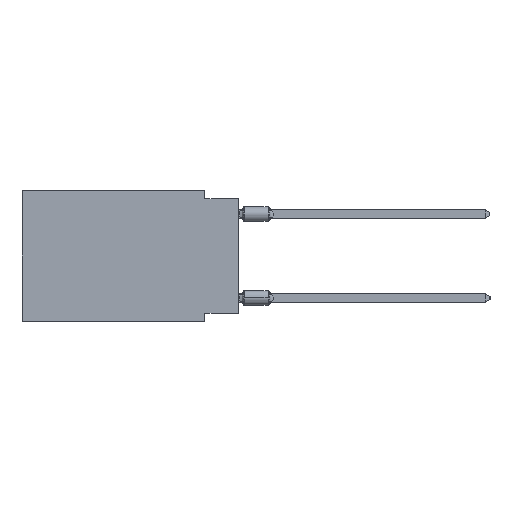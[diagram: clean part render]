
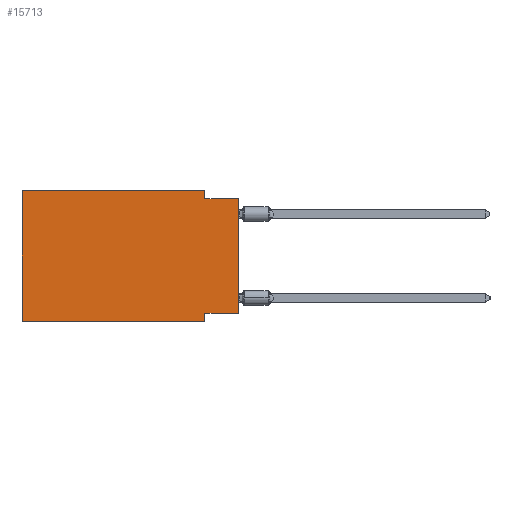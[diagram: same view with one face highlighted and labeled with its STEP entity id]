
A CAD part, left-side view. The second image highlights one B-rep face of the part: STEP entity #15713.
In plain terms, the highlighted planar face has unit normal (-1, 0, 0).
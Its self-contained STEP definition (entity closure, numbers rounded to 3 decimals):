
#450 = EDGE_LOOP ( 'NONE', ( #25573, #35895, #46807, #59695, #64328, #60476, #3902, #8983 ) ) ;
#729 = FACE_OUTER_BOUND ( 'NONE', #450, .T. ) ;
#3515 = AXIS2_PLACEMENT_3D ( 'NONE', #11527, #61065, #20071 ) ;
#3902 = ORIENTED_EDGE ( 'NONE', *, *, #33945, .F. ) ;
#5538 = EDGE_CURVE ( 'NONE', #30922, #60669, #16134, .T. ) ;
#8840 = CARTESIAN_POINT ( 'NONE',  ( 0., 2.54, 0. ) ) ;
#8983 = ORIENTED_EDGE ( 'NONE', *, *, #52530, .F. ) ;
#10487 = VECTOR ( 'NONE', #13177, 1000. ) ;
#11024 = CARTESIAN_POINT ( 'NONE',  ( 0., 16.383, 0. ) ) ;
#11330 = VECTOR ( 'NONE', #32736, 1000. ) ;
#11527 = CARTESIAN_POINT ( 'NONE',  ( 0., 16.383, 0. ) ) ;
#11602 = VERTEX_POINT ( 'NONE', #43726 ) ;
#11729 = LINE ( 'NONE', #26783, #11330 ) ;
#13177 = DIRECTION ( 'NONE',  ( 0., -1., 0. ) ) ;
#13255 = VECTOR ( 'NONE', #61731, 1000. ) ;
#13838 = DIRECTION ( 'NONE',  ( 0., 0., 1. ) ) ;
#14275 = CARTESIAN_POINT ( 'NONE',  ( 0., 2.54, 0. ) ) ;
#15638 = CARTESIAN_POINT ( 'NONE',  ( 0., 2.54, -9.271 ) ) ;
#15713 = ADVANCED_FACE ( 'NONE', ( #729 ), #56473, .F. ) ;
#16100 = DIRECTION ( 'NONE',  ( 0., 1., 0. ) ) ;
#16134 = LINE ( 'NONE', #50898, #13255 ) ;
#18189 = DIRECTION ( 'NONE',  ( 0., -1., 0. ) ) ;
#18984 = LINE ( 'NONE', #8840, #50353 ) ;
#20071 = DIRECTION ( 'NONE',  ( 0., 0., -1. ) ) ;
#20559 = VECTOR ( 'NONE', #16100, 1000. ) ;
#25573 = ORIENTED_EDGE ( 'NONE', *, *, #27191, .T. ) ;
#26417 = CARTESIAN_POINT ( 'NONE',  ( 0., 0., -0.635 ) ) ;
#26783 = CARTESIAN_POINT ( 'NONE',  ( 0., 16.383, 0. ) ) ;
#27191 = EDGE_CURVE ( 'NONE', #29112, #50223, #32538, .T. ) ;
#27917 = LINE ( 'NONE', #46967, #10487 ) ;
#29112 = VERTEX_POINT ( 'NONE', #52447 ) ;
#30400 = VERTEX_POINT ( 'NONE', #49789 ) ;
#30922 = VERTEX_POINT ( 'NONE', #11024 ) ;
#32538 = LINE ( 'NONE', #32864, #53435 ) ;
#32736 = DIRECTION ( 'NONE',  ( 0., 0., 1. ) ) ;
#32851 = EDGE_CURVE ( 'NONE', #30400, #50223, #43091, .T. ) ;
#32864 = CARTESIAN_POINT ( 'NONE',  ( 0., 0., 0. ) ) ;
#33945 = EDGE_CURVE ( 'NONE', #54460, #58143, #37863, .T. ) ;
#35121 = EDGE_CURVE ( 'NONE', #11602, #30922, #11729, .T. ) ;
#35895 = ORIENTED_EDGE ( 'NONE', *, *, #32851, .F. ) ;
#37636 = EDGE_CURVE ( 'NONE', #11602, #58143, #27917, .T. ) ;
#37863 = LINE ( 'NONE', #56621, #49048 ) ;
#38161 = EDGE_CURVE ( 'NONE', #60669, #30400, #18984, .T. ) ;
#42136 = DIRECTION ( 'NONE',  ( 0., 0., -1. ) ) ;
#43091 = LINE ( 'NONE', #63142, #62609 ) ;
#43726 = CARTESIAN_POINT ( 'NONE',  ( 0., 16.383, -9.906 ) ) ;
#46807 = ORIENTED_EDGE ( 'NONE', *, *, #38161, .F. ) ;
#46967 = CARTESIAN_POINT ( 'NONE',  ( 0., 16.383, -9.906 ) ) ;
#49048 = VECTOR ( 'NONE', #42136, 1000. ) ;
#49151 = DIRECTION ( 'NONE',  ( 0., 0., -1. ) ) ;
#49785 = CARTESIAN_POINT ( 'NONE',  ( 0., 2.54, -9.906 ) ) ;
#49789 = CARTESIAN_POINT ( 'NONE',  ( 0., 2.54, -0.635 ) ) ;
#50223 = VERTEX_POINT ( 'NONE', #26417 ) ;
#50353 = VECTOR ( 'NONE', #49151, 1000. ) ;
#50898 = CARTESIAN_POINT ( 'NONE',  ( 0., 16.383, 0. ) ) ;
#52447 = CARTESIAN_POINT ( 'NONE',  ( 0., 0., -9.271 ) ) ;
#52480 = CARTESIAN_POINT ( 'NONE',  ( 0., 0., -9.271 ) ) ;
#52530 = EDGE_CURVE ( 'NONE', #29112, #54460, #61380, .T. ) ;
#53435 = VECTOR ( 'NONE', #13838, 1000. ) ;
#54460 = VERTEX_POINT ( 'NONE', #15638 ) ;
#56473 = PLANE ( 'NONE',  #3515 ) ;
#56621 = CARTESIAN_POINT ( 'NONE',  ( 0., 2.54, -9.906 ) ) ;
#58143 = VERTEX_POINT ( 'NONE', #49785 ) ;
#59695 = ORIENTED_EDGE ( 'NONE', *, *, #5538, .F. ) ;
#60476 = ORIENTED_EDGE ( 'NONE', *, *, #37636, .T. ) ;
#60669 = VERTEX_POINT ( 'NONE', #14275 ) ;
#61065 = DIRECTION ( 'NONE',  ( 1., 0., 0. ) ) ;
#61380 = LINE ( 'NONE', #52480, #20559 ) ;
#61731 = DIRECTION ( 'NONE',  ( 0., -1., 0. ) ) ;
#62609 = VECTOR ( 'NONE', #18189, 1000. ) ;
#63142 = CARTESIAN_POINT ( 'NONE',  ( 0., 0., -0.635 ) ) ;
#64328 = ORIENTED_EDGE ( 'NONE', *, *, #35121, .F. ) ;
